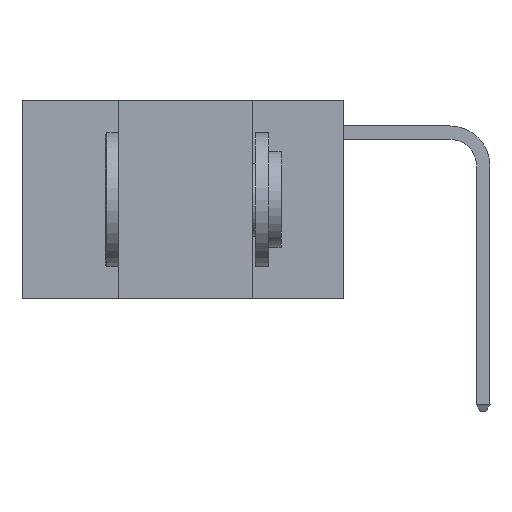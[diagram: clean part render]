
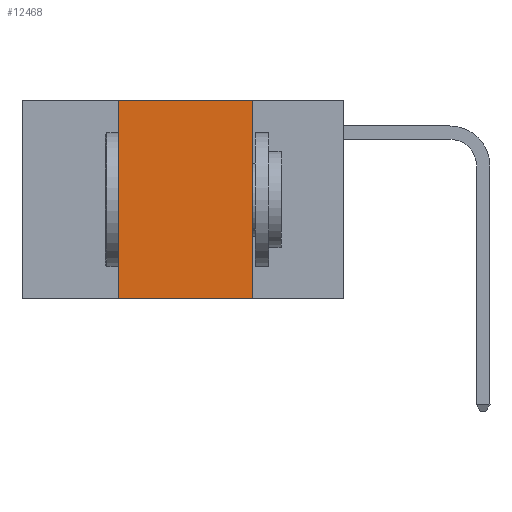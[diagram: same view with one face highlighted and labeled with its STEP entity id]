
A CAD part, left-side view. The second image highlights one B-rep face of the part: STEP entity #12468.
In plain terms, the highlighted planar face has unit normal (-1, 0, 0).
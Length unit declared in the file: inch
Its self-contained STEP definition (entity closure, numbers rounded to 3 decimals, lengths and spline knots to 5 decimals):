
#1083 = ORIENTED_EDGE ( 'NONE', *, *, #17121, .F. ) ;
#1494 = VERTEX_POINT ( 'NONE', #4514 ) ;
#1535 = VECTOR ( 'NONE', #19622, 39.37008 ) ;
#1562 = ORIENTED_EDGE ( 'NONE', *, *, #17171, .T. ) ;
#1693 = VERTEX_POINT ( 'NONE', #5714 ) ;
#1963 = PLANE ( 'NONE',  #6742 ) ;
#2077 = CARTESIAN_POINT ( 'NONE',  ( 0., 0.6, 0. ) ) ;
#2516 = ORIENTED_EDGE ( 'NONE', *, *, #15542, .F. ) ;
#2662 = DIRECTION ( 'NONE',  ( 0., -1., 0. ) ) ;
#2782 = LINE ( 'NONE', #12776, #19680 ) ;
#4226 = LINE ( 'NONE', #7992, #1535 ) ;
#4514 = CARTESIAN_POINT ( 'NONE',  ( 0., 0.42, 0. ) ) ;
#4715 = CARTESIAN_POINT ( 'NONE',  ( 0., 0.17, 0. ) ) ;
#5714 = CARTESIAN_POINT ( 'NONE',  ( 0., 0.42, -0.37 ) ) ;
#6742 = AXIS2_PLACEMENT_3D ( 'NONE', #2077, #17665, #21119 ) ;
#7127 = VERTEX_POINT ( 'NONE', #14605 ) ;
#7992 = CARTESIAN_POINT ( 'NONE',  ( 0., 0.17, 0. ) ) ;
#8646 = DIRECTION ( 'NONE',  ( 0., 0., 1. ) ) ;
#9478 = CARTESIAN_POINT ( 'NONE',  ( 0., 0.6, 0. ) ) ;
#9824 = ORIENTED_EDGE ( 'NONE', *, *, #20168, .F. ) ;
#10534 = LINE ( 'NONE', #18937, #11544 ) ;
#10835 = FACE_OUTER_BOUND ( 'NONE', #18571, .T. ) ;
#11544 = VECTOR ( 'NONE', #8646, 39.37008 ) ;
#12468 = ADVANCED_FACE ( 'NONE', ( #10835 ), #1963, .F. ) ;
#12776 = CARTESIAN_POINT ( 'NONE',  ( 0., 0.6, -0.37 ) ) ;
#14605 = CARTESIAN_POINT ( 'NONE',  ( 0., 0.17, -0.37 ) ) ;
#15542 = EDGE_CURVE ( 'NONE', #1494, #16234, #18205, .T. ) ;
#16234 = VERTEX_POINT ( 'NONE', #4715 ) ;
#17121 = EDGE_CURVE ( 'NONE', #16234, #7127, #4226, .T. ) ;
#17171 = EDGE_CURVE ( 'NONE', #1693, #7127, #2782, .T. ) ;
#17665 = DIRECTION ( 'NONE',  ( 1., 0., 0. ) ) ;
#18205 = LINE ( 'NONE', #9478, #18617 ) ;
#18571 = EDGE_LOOP ( 'NONE', ( #1083, #2516, #9824, #1562 ) ) ;
#18617 = VECTOR ( 'NONE', #19753, 39.37008 ) ;
#18937 = CARTESIAN_POINT ( 'NONE',  ( 0., 0.42, 0. ) ) ;
#19622 = DIRECTION ( 'NONE',  ( 0., 0., -1. ) ) ;
#19680 = VECTOR ( 'NONE', #2662, 39.37008 ) ;
#19753 = DIRECTION ( 'NONE',  ( 0., -1., 0. ) ) ;
#20168 = EDGE_CURVE ( 'NONE', #1693, #1494, #10534, .T. ) ;
#21119 = DIRECTION ( 'NONE',  ( 0., 0., -1. ) ) ;
